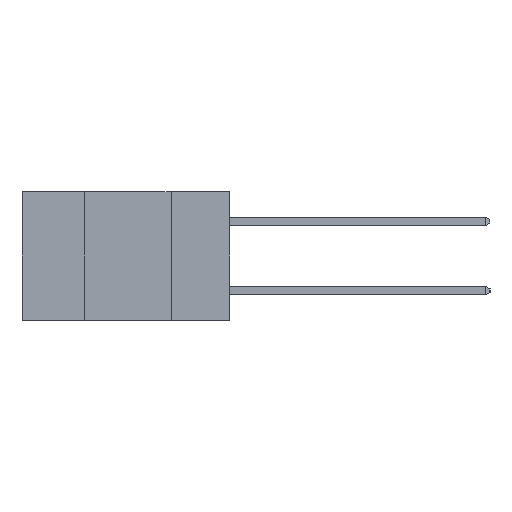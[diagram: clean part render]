
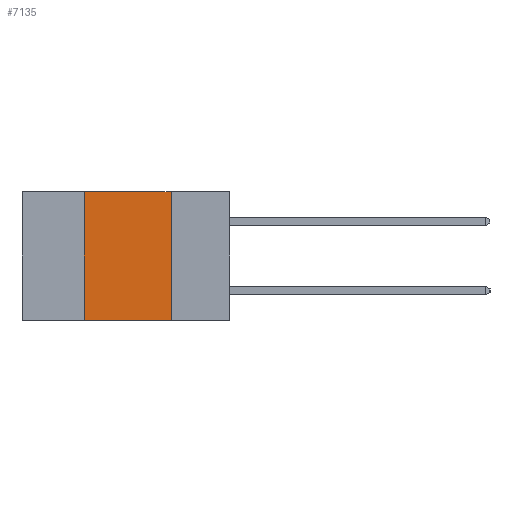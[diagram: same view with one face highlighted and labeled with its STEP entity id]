
A CAD part, left-side view. The second image highlights one B-rep face of the part: STEP entity #7135.
In plain terms, the highlighted planar face has unit normal (-1, 0, 0).
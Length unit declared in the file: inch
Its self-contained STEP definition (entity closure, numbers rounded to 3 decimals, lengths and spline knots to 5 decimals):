
#517 = EDGE_CURVE ( 'NONE', #2797, #2205, #4593, .T. ) ;
#561 = CARTESIAN_POINT ( 'NONE',  ( 0., 0.6, -0.37 ) ) ;
#599 = CARTESIAN_POINT ( 'NONE',  ( 0., 0.17, -0.37 ) ) ;
#654 = PLANE ( 'NONE',  #8647 ) ;
#1572 = LINE ( 'NONE', #6775, #3750 ) ;
#1632 = VECTOR ( 'NONE', #7618, 39.37008 ) ;
#1740 = VERTEX_POINT ( 'NONE', #2607 ) ;
#1784 = VECTOR ( 'NONE', #8843, 39.37008 ) ;
#2099 = CARTESIAN_POINT ( 'NONE',  ( 0., 0.42, -0.37 ) ) ;
#2205 = VERTEX_POINT ( 'NONE', #7276 ) ;
#2372 = EDGE_CURVE ( 'NONE', #2797, #2927, #10139, .T. ) ;
#2607 = CARTESIAN_POINT ( 'NONE',  ( 0., 0.17, 0. ) ) ;
#2742 = CARTESIAN_POINT ( 'NONE',  ( 0., 0.42, 0. ) ) ;
#2797 = VERTEX_POINT ( 'NONE', #3936 ) ;
#2927 = VERTEX_POINT ( 'NONE', #2742 ) ;
#3523 = EDGE_LOOP ( 'NONE', ( #9973, #5904, #5176, #8405 ) ) ;
#3750 = VECTOR ( 'NONE', #9869, 39.37008 ) ;
#3910 = DIRECTION ( 'NONE',  ( 0., 0., -1. ) ) ;
#3936 = CARTESIAN_POINT ( 'NONE',  ( 0., 0.42, -0.37 ) ) ;
#4593 = LINE ( 'NONE', #561, #1784 ) ;
#5176 = ORIENTED_EDGE ( 'NONE', *, *, #2372, .F. ) ;
#5308 = DIRECTION ( 'NONE',  ( 0., 0., -1. ) ) ;
#5904 = ORIENTED_EDGE ( 'NONE', *, *, #9832, .F. ) ;
#6775 = CARTESIAN_POINT ( 'NONE',  ( 0., 0.6, 0. ) ) ;
#6870 = LINE ( 'NONE', #599, #9724 ) ;
#7135 = ADVANCED_FACE ( 'NONE', ( #7562 ), #654, .F. ) ;
#7276 = CARTESIAN_POINT ( 'NONE',  ( 0., 0.17, -0.37 ) ) ;
#7562 = FACE_OUTER_BOUND ( 'NONE', #3523, .T. ) ;
#7618 = DIRECTION ( 'NONE',  ( 0., 0., 1. ) ) ;
#8405 = ORIENTED_EDGE ( 'NONE', *, *, #517, .T. ) ;
#8534 = DIRECTION ( 'NONE',  ( 1., 0., 0. ) ) ;
#8647 = AXIS2_PLACEMENT_3D ( 'NONE', #9375, #8534, #3910 ) ;
#8843 = DIRECTION ( 'NONE',  ( 0., -1., 0. ) ) ;
#9375 = CARTESIAN_POINT ( 'NONE',  ( 0., 0.6, 0. ) ) ;
#9724 = VECTOR ( 'NONE', #5308, 39.37008 ) ;
#9832 = EDGE_CURVE ( 'NONE', #2927, #1740, #1572, .T. ) ;
#9869 = DIRECTION ( 'NONE',  ( 0., -1., 0. ) ) ;
#9973 = ORIENTED_EDGE ( 'NONE', *, *, #10010, .F. ) ;
#10010 = EDGE_CURVE ( 'NONE', #1740, #2205, #6870, .T. ) ;
#10139 = LINE ( 'NONE', #2099, #1632 ) ;
